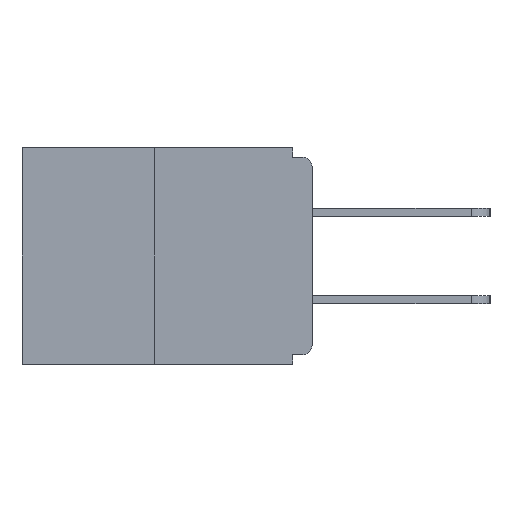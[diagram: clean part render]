
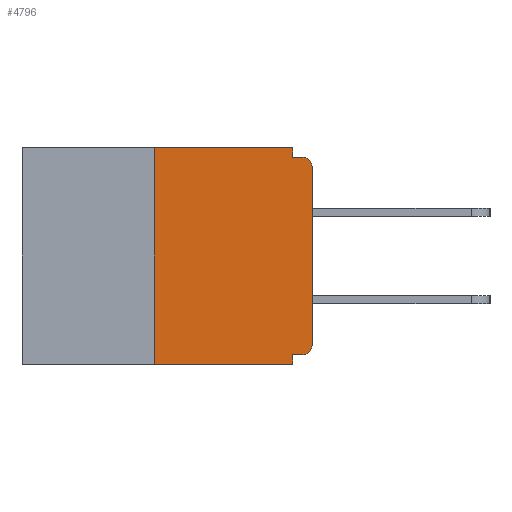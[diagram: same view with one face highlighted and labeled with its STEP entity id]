
A CAD part, left-side view. The second image highlights one B-rep face of the part: STEP entity #4796.
In plain terms, the highlighted planar face has unit normal (-1, 0, 0).
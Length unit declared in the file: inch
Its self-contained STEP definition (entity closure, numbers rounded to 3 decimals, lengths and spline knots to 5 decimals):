
#6 = LINE ( 'NONE', #24591, #13441 ) ;
#102 = VERTEX_POINT ( 'NONE', #24799 ) ;
#943 = AXIS2_PLACEMENT_3D ( 'NONE', #15735, #22385, #4616 ) ;
#1630 = CARTESIAN_POINT ( 'NONE',  ( 0., 0.46, 0. ) ) ;
#1967 = ORIENTED_EDGE ( 'NONE', *, *, #2558, .T. ) ;
#2287 = LINE ( 'NONE', #3341, #27488 ) ;
#2558 = EDGE_CURVE ( 'NONE', #10488, #20912, #5131, .T. ) ;
#2631 = VECTOR ( 'NONE', #19692, 39.37008 ) ;
#3341 = CARTESIAN_POINT ( 'NONE',  ( 0., 0.031, 0. ) ) ;
#3495 = DIRECTION ( 'NONE',  ( 0., -1., 0. ) ) ;
#4616 = DIRECTION ( 'NONE',  ( 0., 0., -1. ) ) ;
#4786 = FACE_OUTER_BOUND ( 'NONE', #15576, .T. ) ;
#4796 = ADVANCED_FACE ( 'NONE', ( #4786 ), #15536, .F. ) ;
#4913 = DIRECTION ( 'NONE',  ( -1., 0., 0. ) ) ;
#5131 = LINE ( 'NONE', #6369, #23253 ) ;
#5147 = EDGE_CURVE ( 'NONE', #102, #9941, #12615, .T. ) ;
#5551 = EDGE_CURVE ( 'NONE', #16969, #102, #2287, .T. ) ;
#6369 = CARTESIAN_POINT ( 'NONE',  ( 0., 0., 0. ) ) ;
#6488 = EDGE_CURVE ( 'NONE', #20805, #12452, #10411, .T. ) ;
#6839 = LINE ( 'NONE', #1630, #17481 ) ;
#6867 = CARTESIAN_POINT ( 'NONE',  ( 0., 0.25, -0.343 ) ) ;
#7550 = ORIENTED_EDGE ( 'NONE', *, *, #6488, .F. ) ;
#7857 = VECTOR ( 'NONE', #16891, 39.37008 ) ;
#8186 = AXIS2_PLACEMENT_3D ( 'NONE', #8910, #22689, #17720 ) ;
#8771 = ORIENTED_EDGE ( 'NONE', *, *, #5147, .F. ) ;
#8910 = CARTESIAN_POINT ( 'NONE',  ( 0., 0.015, -0.03 ) ) ;
#9371 = LINE ( 'NONE', #17672, #2631 ) ;
#9941 = VERTEX_POINT ( 'NONE', #11427 ) ;
#10411 = LINE ( 'NONE', #27348, #24558 ) ;
#10488 = VERTEX_POINT ( 'NONE', #21119 ) ;
#11427 = CARTESIAN_POINT ( 'NONE',  ( 0., 0.015, -0.015 ) ) ;
#12070 = VERTEX_POINT ( 'NONE', #18288 ) ;
#12377 = CARTESIAN_POINT ( 'NONE',  ( 0., 0., -0.328 ) ) ;
#12452 = VERTEX_POINT ( 'NONE', #17012 ) ;
#12494 = DIRECTION ( 'NONE',  ( 0., 0., -1. ) ) ;
#12599 = AXIS2_PLACEMENT_3D ( 'NONE', #18314, #4913, #25371 ) ;
#12615 = LINE ( 'NONE', #15073, #17561 ) ;
#13069 = DIRECTION ( 'NONE',  ( 0., 0., -1. ) ) ;
#13441 = VECTOR ( 'NONE', #13069, 39.37008 ) ;
#14191 = CARTESIAN_POINT ( 'NONE',  ( 0., 0., -0.03 ) ) ;
#15073 = CARTESIAN_POINT ( 'NONE',  ( 0., 0., -0.015 ) ) ;
#15536 = PLANE ( 'NONE',  #943 ) ;
#15576 = EDGE_LOOP ( 'NONE', ( #28916, #7550, #18148, #17779, #17174, #20978, #1967, #19102, #8771, #21625 ) ) ;
#15735 = CARTESIAN_POINT ( 'NONE',  ( 0., 0.46, 0. ) ) ;
#16029 = EDGE_CURVE ( 'NONE', #20805, #18388, #9371, .T. ) ;
#16134 = CIRCLE ( 'NONE', #8186, 0.015 ) ;
#16298 = EDGE_CURVE ( 'NONE', #24825, #18388, #6, .T. ) ;
#16405 = DIRECTION ( 'NONE',  ( 0., 0., 1. ) ) ;
#16891 = DIRECTION ( 'NONE',  ( 0., 1., 0. ) ) ;
#16969 = VERTEX_POINT ( 'NONE', #24052 ) ;
#17012 = CARTESIAN_POINT ( 'NONE',  ( 0., 0.25, 0. ) ) ;
#17174 = ORIENTED_EDGE ( 'NONE', *, *, #21423, .F. ) ;
#17481 = VECTOR ( 'NONE', #3495, 39.37008 ) ;
#17561 = VECTOR ( 'NONE', #26388, 39.37008 ) ;
#17672 = CARTESIAN_POINT ( 'NONE',  ( 0., 0.46, -0.343 ) ) ;
#17720 = DIRECTION ( 'NONE',  ( 0., 0., -1. ) ) ;
#17779 = ORIENTED_EDGE ( 'NONE', *, *, #16298, .F. ) ;
#18148 = ORIENTED_EDGE ( 'NONE', *, *, #16029, .T. ) ;
#18176 = DIRECTION ( 'NONE',  ( 0., 0., 1. ) ) ;
#18288 = CARTESIAN_POINT ( 'NONE',  ( 0., 0.015, -0.328 ) ) ;
#18314 = CARTESIAN_POINT ( 'NONE',  ( 0., 0.015, -0.313 ) ) ;
#18388 = VERTEX_POINT ( 'NONE', #26949 ) ;
#19102 = ORIENTED_EDGE ( 'NONE', *, *, #26123, .T. ) ;
#19692 = DIRECTION ( 'NONE',  ( 0., -1., 0. ) ) ;
#19909 = LINE ( 'NONE', #12377, #7857 ) ;
#20805 = VERTEX_POINT ( 'NONE', #6867 ) ;
#20912 = VERTEX_POINT ( 'NONE', #14191 ) ;
#20978 = ORIENTED_EDGE ( 'NONE', *, *, #26193, .T. ) ;
#21119 = CARTESIAN_POINT ( 'NONE',  ( 0., 0., -0.313 ) ) ;
#21423 = EDGE_CURVE ( 'NONE', #12070, #24825, #19909, .T. ) ;
#21478 = CIRCLE ( 'NONE', #12599, 0.015 ) ;
#21625 = ORIENTED_EDGE ( 'NONE', *, *, #5551, .F. ) ;
#22385 = DIRECTION ( 'NONE',  ( 1., 0., 0. ) ) ;
#22689 = DIRECTION ( 'NONE',  ( -1., 0., 0. ) ) ;
#23253 = VECTOR ( 'NONE', #18176, 39.37008 ) ;
#24016 = CARTESIAN_POINT ( 'NONE',  ( 0., 0.031, -0.328 ) ) ;
#24052 = CARTESIAN_POINT ( 'NONE',  ( 0., 0.031, 0. ) ) ;
#24558 = VECTOR ( 'NONE', #16405, 39.37008 ) ;
#24591 = CARTESIAN_POINT ( 'NONE',  ( 0., 0.031, -0.343 ) ) ;
#24799 = CARTESIAN_POINT ( 'NONE',  ( 0., 0.031, -0.015 ) ) ;
#24825 = VERTEX_POINT ( 'NONE', #24016 ) ;
#25371 = DIRECTION ( 'NONE',  ( 0., 0., -1. ) ) ;
#26123 = EDGE_CURVE ( 'NONE', #20912, #9941, #16134, .T. ) ;
#26193 = EDGE_CURVE ( 'NONE', #12070, #10488, #21478, .T. ) ;
#26388 = DIRECTION ( 'NONE',  ( 0., -1., 0. ) ) ;
#26949 = CARTESIAN_POINT ( 'NONE',  ( 0., 0.031, -0.343 ) ) ;
#27348 = CARTESIAN_POINT ( 'NONE',  ( 0., 0.25, 0. ) ) ;
#27488 = VECTOR ( 'NONE', #12494, 39.37008 ) ;
#28330 = EDGE_CURVE ( 'NONE', #12452, #16969, #6839, .T. ) ;
#28916 = ORIENTED_EDGE ( 'NONE', *, *, #28330, .F. ) ;
